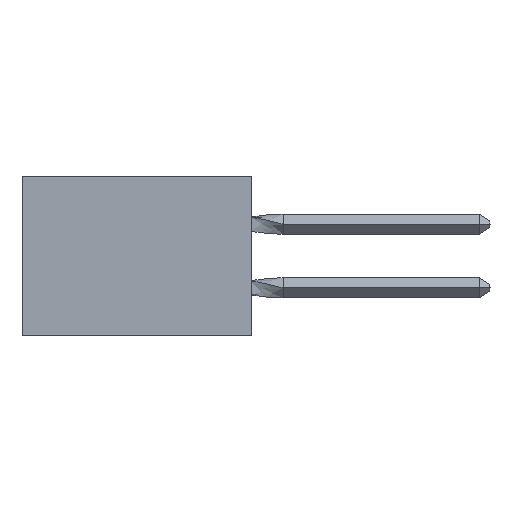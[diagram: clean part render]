
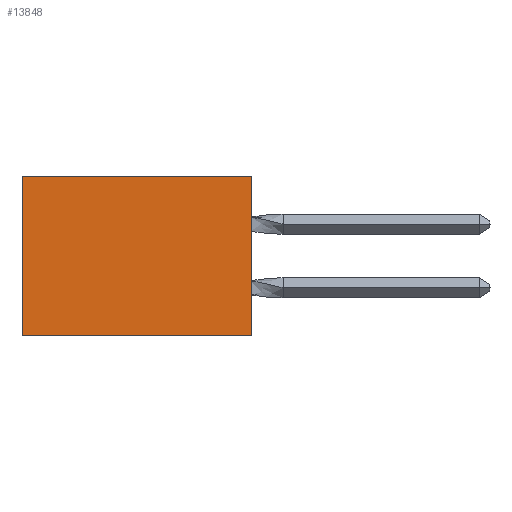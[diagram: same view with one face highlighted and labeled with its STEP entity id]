
A CAD part, left-side view. The second image highlights one B-rep face of the part: STEP entity #13848.
In plain terms, the highlighted planar face has unit normal (-1, 0, 0).
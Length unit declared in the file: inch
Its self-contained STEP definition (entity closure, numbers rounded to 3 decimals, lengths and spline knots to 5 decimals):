
#151 = VERTEX_POINT ( 'NONE', #12152 ) ;
#1696 = EDGE_CURVE ( 'NONE', #25720, #8366, #29278, .T. ) ;
#3701 = CARTESIAN_POINT ( 'NONE',  ( 0.305, 0., -0.5 ) ) ;
#4691 = EDGE_CURVE ( 'NONE', #151, #8904, #7475, .T. ) ;
#5665 = CARTESIAN_POINT ( 'NONE',  ( 0.305, 0., 0. ) ) ;
#7272 = VECTOR ( 'NONE', #27428, 39.37008 ) ;
#7475 = LINE ( 'NONE', #3701, #35195 ) ;
#7741 = PLANE ( 'NONE',  #20562 ) ;
#7854 = DIRECTION ( 'NONE',  ( 0., 0., -1. ) ) ;
#8344 = ORIENTED_EDGE ( 'NONE', *, *, #1696, .T. ) ;
#8366 = VERTEX_POINT ( 'NONE', #15143 ) ;
#8904 = VERTEX_POINT ( 'NONE', #20233 ) ;
#9153 = DIRECTION ( 'NONE',  ( 0., 1., 0. ) ) ;
#9924 = ORIENTED_EDGE ( 'NONE', *, *, #4691, .F. ) ;
#12152 = CARTESIAN_POINT ( 'NONE',  ( 0.305, 0., -0.5 ) ) ;
#13153 = VECTOR ( 'NONE', #35471, 39.37008 ) ;
#13418 = EDGE_LOOP ( 'NONE', ( #34996, #9924, #27504, #8344 ) ) ;
#13848 = ADVANCED_FACE ( 'NONE', ( #19824 ), #7741, .F. ) ;
#14626 = LINE ( 'NONE', #21150, #7272 ) ;
#14779 = EDGE_CURVE ( 'NONE', #8366, #8904, #14626, .T. ) ;
#15143 = CARTESIAN_POINT ( 'NONE',  ( 0.305, 0.72, 0. ) ) ;
#19824 = FACE_OUTER_BOUND ( 'NONE', #13418, .T. ) ;
#20233 = CARTESIAN_POINT ( 'NONE',  ( 0.305, 0.72, -0.5 ) ) ;
#20562 = AXIS2_PLACEMENT_3D ( 'NONE', #29864, #21596, #7854 ) ;
#21150 = CARTESIAN_POINT ( 'NONE',  ( 0.305, 0.72, -0.5 ) ) ;
#21596 = DIRECTION ( 'NONE',  ( 1., 0., 0. ) ) ;
#23086 = LINE ( 'NONE', #26807, #13153 ) ;
#23465 = DIRECTION ( 'NONE',  ( 0., 1., 0. ) ) ;
#25491 = EDGE_CURVE ( 'NONE', #25720, #151, #23086, .T. ) ;
#25720 = VERTEX_POINT ( 'NONE', #5665 ) ;
#26677 = CARTESIAN_POINT ( 'NONE',  ( 0.305, 0., 0. ) ) ;
#26807 = CARTESIAN_POINT ( 'NONE',  ( 0.305, 0., -0.5 ) ) ;
#27428 = DIRECTION ( 'NONE',  ( 0., 0., -1. ) ) ;
#27504 = ORIENTED_EDGE ( 'NONE', *, *, #25491, .F. ) ;
#29278 = LINE ( 'NONE', #26677, #34948 ) ;
#29864 = CARTESIAN_POINT ( 'NONE',  ( 0.305, 0., -0.5 ) ) ;
#34948 = VECTOR ( 'NONE', #23465, 39.37008 ) ;
#34996 = ORIENTED_EDGE ( 'NONE', *, *, #14779, .T. ) ;
#35195 = VECTOR ( 'NONE', #9153, 39.37008 ) ;
#35471 = DIRECTION ( 'NONE',  ( 0., 0., -1. ) ) ;
